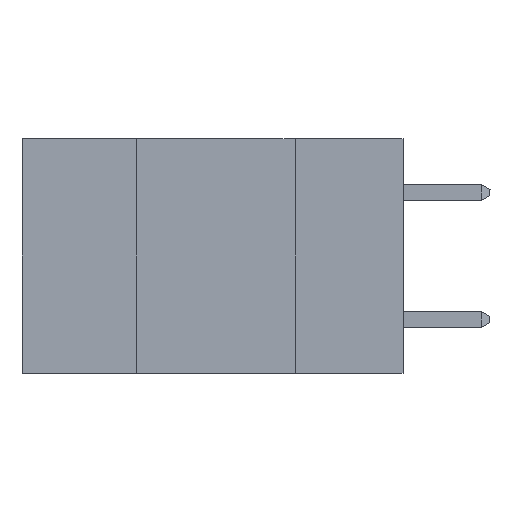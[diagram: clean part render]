
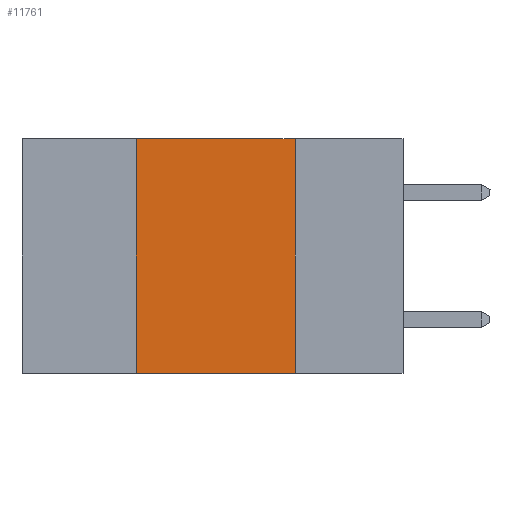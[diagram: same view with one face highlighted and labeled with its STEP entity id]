
A CAD part, left-side view. The second image highlights one B-rep face of the part: STEP entity #11761.
In plain terms, the highlighted planar face has unit normal (-1, 0, 0).
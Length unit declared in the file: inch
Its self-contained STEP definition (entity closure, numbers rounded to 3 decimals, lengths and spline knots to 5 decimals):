
#153 = DIRECTION ( 'NONE',  ( 0., -1., 0. ) ) ;
#237 = LINE ( 'NONE', #10013, #13742 ) ;
#778 = VERTEX_POINT ( 'NONE', #1031 ) ;
#860 = CARTESIAN_POINT ( 'NONE',  ( 0., 0.6, 0. ) ) ;
#1031 = CARTESIAN_POINT ( 'NONE',  ( 0., 0.17, -0.37 ) ) ;
#1306 = CARTESIAN_POINT ( 'NONE',  ( 0., 0.17, 0. ) ) ;
#2197 = ORIENTED_EDGE ( 'NONE', *, *, #14105, .T. ) ;
#2465 = LINE ( 'NONE', #2828, #10711 ) ;
#2681 = CARTESIAN_POINT ( 'NONE',  ( 0., 0.6, -0.37 ) ) ;
#2828 = CARTESIAN_POINT ( 'NONE',  ( 0., 0.42, 0. ) ) ;
#3511 = ORIENTED_EDGE ( 'NONE', *, *, #20825, .F. ) ;
#4402 = DIRECTION ( 'NONE',  ( 1., 0., 0. ) ) ;
#4673 = VERTEX_POINT ( 'NONE', #12385 ) ;
#5777 = EDGE_CURVE ( 'NONE', #4673, #10969, #2465, .T. ) ;
#5830 = VECTOR ( 'NONE', #153, 39.37008 ) ;
#7651 = CARTESIAN_POINT ( 'NONE',  ( 0., 0.42, 0. ) ) ;
#8563 = VECTOR ( 'NONE', #14920, 39.37008 ) ;
#8990 = CARTESIAN_POINT ( 'NONE',  ( 0., 0.6, 0. ) ) ;
#10013 = CARTESIAN_POINT ( 'NONE',  ( 0., 0.17, 0. ) ) ;
#10711 = VECTOR ( 'NONE', #16882, 39.37008 ) ;
#10969 = VERTEX_POINT ( 'NONE', #7651 ) ;
#11761 = ADVANCED_FACE ( 'NONE', ( #19572 ), #14942, .F. ) ;
#12385 = CARTESIAN_POINT ( 'NONE',  ( 0., 0.42, -0.37 ) ) ;
#13305 = AXIS2_PLACEMENT_3D ( 'NONE', #860, #4402, #16669 ) ;
#13742 = VECTOR ( 'NONE', #17032, 39.37008 ) ;
#14105 = EDGE_CURVE ( 'NONE', #4673, #778, #22388, .T. ) ;
#14495 = EDGE_CURVE ( 'NONE', #10969, #16124, #19221, .T. ) ;
#14920 = DIRECTION ( 'NONE',  ( 0., -1., 0. ) ) ;
#14942 = PLANE ( 'NONE',  #13305 ) ;
#16124 = VERTEX_POINT ( 'NONE', #1306 ) ;
#16669 = DIRECTION ( 'NONE',  ( 0., 0., -1. ) ) ;
#16729 = ORIENTED_EDGE ( 'NONE', *, *, #5777, .F. ) ;
#16882 = DIRECTION ( 'NONE',  ( 0., 0., 1. ) ) ;
#17032 = DIRECTION ( 'NONE',  ( 0., 0., -1. ) ) ;
#19221 = LINE ( 'NONE', #8990, #5830 ) ;
#19572 = FACE_OUTER_BOUND ( 'NONE', #21767, .T. ) ;
#19684 = ORIENTED_EDGE ( 'NONE', *, *, #14495, .F. ) ;
#20825 = EDGE_CURVE ( 'NONE', #16124, #778, #237, .T. ) ;
#21767 = EDGE_LOOP ( 'NONE', ( #3511, #19684, #16729, #2197 ) ) ;
#22388 = LINE ( 'NONE', #2681, #8563 ) ;
